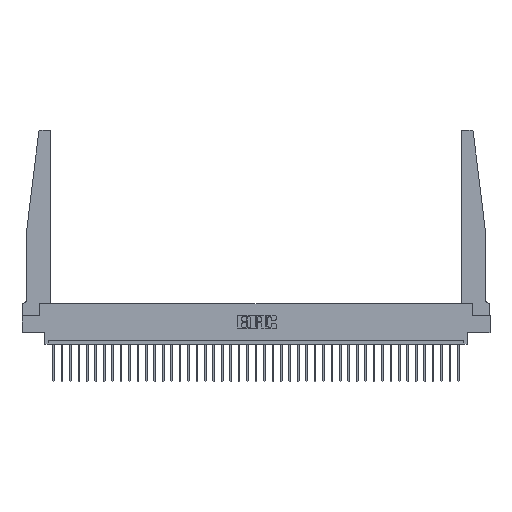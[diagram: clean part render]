
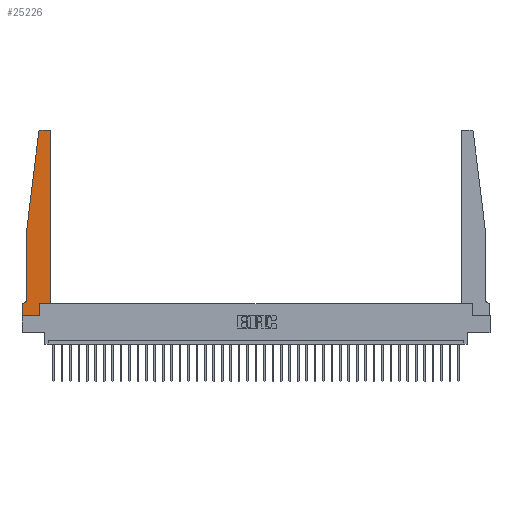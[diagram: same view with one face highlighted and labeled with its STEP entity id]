
A CAD part, top view. The second image highlights one B-rep face of the part: STEP entity #25226.
In plain terms, the highlighted planar face has unit normal (0, 0, 1).
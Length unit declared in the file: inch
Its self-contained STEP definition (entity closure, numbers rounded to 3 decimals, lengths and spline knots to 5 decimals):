
#275 = LINE ( 'NONE', #24407, #17898 ) ;
#472 = ORIENTED_EDGE ( 'NONE', *, *, #25737, .T. ) ;
#1003 = CARTESIAN_POINT ( 'NONE',  ( 0.015, 0.1875, 0.37 ) ) ;
#1305 = EDGE_CURVE ( 'NONE', #15620, #22994, #7373, .T. ) ;
#1400 = DIRECTION ( 'NONE',  ( 1., 0., 0. ) ) ;
#2108 = CARTESIAN_POINT ( 'NONE',  ( 0.2605, 0., 0.37 ) ) ;
#2264 = EDGE_CURVE ( 'NONE', #9354, #15620, #12576, .T. ) ;
#2309 = ORIENTED_EDGE ( 'NONE', *, *, #21912, .T. ) ;
#2350 = CARTESIAN_POINT ( 'NONE',  ( 0.015, 0.2375, 0.37 ) ) ;
#2452 = AXIS2_PLACEMENT_3D ( 'NONE', #12494, #7566, #12851 ) ;
#2934 = LINE ( 'NONE', #13677, #27697 ) ;
#2964 = CARTESIAN_POINT ( 'NONE',  ( 0.2605, 0.18, 0.37 ) ) ;
#3430 = EDGE_CURVE ( 'NONE', #22924, #13475, #25463, .T. ) ;
#3601 = CARTESIAN_POINT ( 'NONE',  ( 0., 0.1875, 0.37 ) ) ;
#3640 = DIRECTION ( 'NONE',  ( 1., 0., 0. ) ) ;
#4066 = ORIENTED_EDGE ( 'NONE', *, *, #1305, .T. ) ;
#4164 = DIRECTION ( 'NONE',  ( 1., 0., 0. ) ) ;
#4572 = VERTEX_POINT ( 'NONE', #10704 ) ;
#5088 = DIRECTION ( 'NONE',  ( -1., 0., 0. ) ) ;
#5857 = AXIS2_PLACEMENT_3D ( 'NONE', #12297, #9497, #1400 ) ;
#6456 = CARTESIAN_POINT ( 'NONE',  ( 0.425, 0.18, 0.37 ) ) ;
#6705 = CARTESIAN_POINT ( 'NONE',  ( 0., 0., 0.37 ) ) ;
#7014 = VERTEX_POINT ( 'NONE', #6705 ) ;
#7111 = VERTEX_POINT ( 'NONE', #2108 ) ;
#7113 = EDGE_CURVE ( 'NONE', #25259, #32412, #34349, .T. ) ;
#7373 = LINE ( 'NONE', #18121, #11599 ) ;
#7566 = DIRECTION ( 'NONE',  ( 0., 0., 1. ) ) ;
#9354 = VERTEX_POINT ( 'NONE', #29166 ) ;
#9384 = CARTESIAN_POINT ( 'NONE',  ( 0.065, 1.25, 0.37 ) ) ;
#9497 = DIRECTION ( 'NONE',  ( 0., 0., 1. ) ) ;
#9961 = EDGE_CURVE ( 'NONE', #7014, #7111, #21702, .T. ) ;
#10303 = DIRECTION ( 'NONE',  ( 0., -1., 0. ) ) ;
#10604 = ORIENTED_EDGE ( 'NONE', *, *, #29707, .T. ) ;
#10704 = CARTESIAN_POINT ( 'NONE',  ( 0.065, 0.2375, 0.37 ) ) ;
#11116 = CARTESIAN_POINT ( 'NONE',  ( 0.24675, 2.72367, 0.37 ) ) ;
#11327 = AXIS2_PLACEMENT_3D ( 'NONE', #2350, #17845, #23849 ) ;
#11599 = VECTOR ( 'NONE', #5088, 39.37008 ) ;
#11705 = VECTOR ( 'NONE', #10303, 39.37008 ) ;
#11904 = CARTESIAN_POINT ( 'NONE',  ( 0.425, 0.18, 0.37 ) ) ;
#12297 = CARTESIAN_POINT ( 'NONE',  ( 0.395, 2.72, 0.37 ) ) ;
#12494 = CARTESIAN_POINT ( 'NONE',  ( 0.27653, 2.72, 0.37 ) ) ;
#12576 = CIRCLE ( 'NONE', #5857, 0.03 ) ;
#12851 = DIRECTION ( 'NONE',  ( 1., 0., 0. ) ) ;
#13249 = VECTOR ( 'NONE', #28291, 39.37008 ) ;
#13475 = VERTEX_POINT ( 'NONE', #9384 ) ;
#13570 = ORIENTED_EDGE ( 'NONE', *, *, #7113, .T. ) ;
#13677 = CARTESIAN_POINT ( 'NONE',  ( 0.2605, 0.18, 0.37 ) ) ;
#14848 = EDGE_CURVE ( 'NONE', #22994, #22924, #17626, .T. ) ;
#15304 = DIRECTION ( 'NONE',  ( -1., 0., 0. ) ) ;
#15620 = VERTEX_POINT ( 'NONE', #25648 ) ;
#16400 = CARTESIAN_POINT ( 'NONE',  ( 0., 0., 0.37 ) ) ;
#16460 = DIRECTION ( 'NONE',  ( 0., -1., 0. ) ) ;
#16493 = DIRECTION ( 'NONE',  ( 0., 1., 0. ) ) ;
#16607 = EDGE_CURVE ( 'NONE', #24703, #9354, #22484, .T. ) ;
#16753 = ORIENTED_EDGE ( 'NONE', *, *, #3430, .T. ) ;
#17626 = CIRCLE ( 'NONE', #2452, 0.03 ) ;
#17845 = DIRECTION ( 'NONE',  ( 0., 0., -1. ) ) ;
#17898 = VECTOR ( 'NONE', #16460, 39.37008 ) ;
#18121 = CARTESIAN_POINT ( 'NONE',  ( 0.25, 2.75, 0.37 ) ) ;
#18236 = CARTESIAN_POINT ( 'NONE',  ( 0., 0., 0.37 ) ) ;
#18675 = VERTEX_POINT ( 'NONE', #2964 ) ;
#19661 = ORIENTED_EDGE ( 'NONE', *, *, #9961, .T. ) ;
#19781 = ORIENTED_EDGE ( 'NONE', *, *, #16607, .T. ) ;
#20371 = ORIENTED_EDGE ( 'NONE', *, *, #22022, .T. ) ;
#21702 = LINE ( 'NONE', #16400, #24401 ) ;
#21910 = ORIENTED_EDGE ( 'NONE', *, *, #30681, .T. ) ;
#21912 = EDGE_CURVE ( 'NONE', #32412, #7014, #34455, .T. ) ;
#22006 = AXIS2_PLACEMENT_3D ( 'NONE', #25326, #33584, #4164 ) ;
#22022 = EDGE_CURVE ( 'NONE', #13475, #4572, #275, .T. ) ;
#22265 = VECTOR ( 'NONE', #15304, 39.37008 ) ;
#22330 = ORIENTED_EDGE ( 'NONE', *, *, #2264, .T. ) ;
#22484 = LINE ( 'NONE', #6456, #13249 ) ;
#22924 = VERTEX_POINT ( 'NONE', #11116 ) ;
#22994 = VERTEX_POINT ( 'NONE', #29814 ) ;
#23849 = DIRECTION ( 'NONE',  ( -1., 0., 0. ) ) ;
#24401 = VECTOR ( 'NONE', #32977, 39.37008 ) ;
#24407 = CARTESIAN_POINT ( 'NONE',  ( 0.065, 1.25, 0.37 ) ) ;
#24703 = VERTEX_POINT ( 'NONE', #30170 ) ;
#25226 = ADVANCED_FACE ( 'NONE', ( #25669 ), #30965, .T. ) ;
#25259 = VERTEX_POINT ( 'NONE', #1003 ) ;
#25326 = CARTESIAN_POINT ( 'NONE',  ( 0., 0.1875, 0.37 ) ) ;
#25463 = LINE ( 'NONE', #27918, #31576 ) ;
#25632 = DIRECTION ( 'NONE',  ( -0.122, -0.992, 0. ) ) ;
#25648 = CARTESIAN_POINT ( 'NONE',  ( 0.395, 2.75, 0.37 ) ) ;
#25669 = FACE_OUTER_BOUND ( 'NONE', #34229, .T. ) ;
#25737 = EDGE_CURVE ( 'NONE', #4572, #25259, #28798, .T. ) ;
#26742 = ORIENTED_EDGE ( 'NONE', *, *, #14848, .T. ) ;
#27697 = VECTOR ( 'NONE', #16493, 39.37008 ) ;
#27918 = CARTESIAN_POINT ( 'NONE',  ( 0.065, 1.25, 0.37 ) ) ;
#28291 = DIRECTION ( 'NONE',  ( 0., 1., 0. ) ) ;
#28718 = CARTESIAN_POINT ( 'NONE',  ( 0.065, 0.1875, 0.37 ) ) ;
#28798 = CIRCLE ( 'NONE', #11327, 0.05 ) ;
#29166 = CARTESIAN_POINT ( 'NONE',  ( 0.425, 2.72, 0.37 ) ) ;
#29468 = VECTOR ( 'NONE', #3640, 39.37008 ) ;
#29707 = EDGE_CURVE ( 'NONE', #7111, #18675, #2934, .T. ) ;
#29814 = CARTESIAN_POINT ( 'NONE',  ( 0.27653, 2.75, 0.37 ) ) ;
#30170 = CARTESIAN_POINT ( 'NONE',  ( 0.425, 0.18, 0.37 ) ) ;
#30681 = EDGE_CURVE ( 'NONE', #18675, #24703, #33075, .T. ) ;
#30965 = PLANE ( 'NONE',  #22006 ) ;
#31576 = VECTOR ( 'NONE', #25632, 39.37008 ) ;
#32412 = VERTEX_POINT ( 'NONE', #3601 ) ;
#32977 = DIRECTION ( 'NONE',  ( 1., 0., 0. ) ) ;
#33075 = LINE ( 'NONE', #11904, #29468 ) ;
#33584 = DIRECTION ( 'NONE',  ( 0., 0., 1. ) ) ;
#34229 = EDGE_LOOP ( 'NONE', ( #4066, #26742, #16753, #20371, #472, #13570, #2309, #19661, #10604, #21910, #19781, #22330 ) ) ;
#34349 = LINE ( 'NONE', #28718, #22265 ) ;
#34455 = LINE ( 'NONE', #18236, #11705 ) ;
